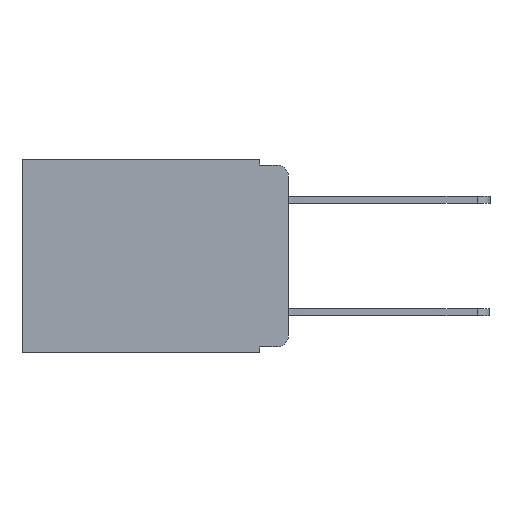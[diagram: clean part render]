
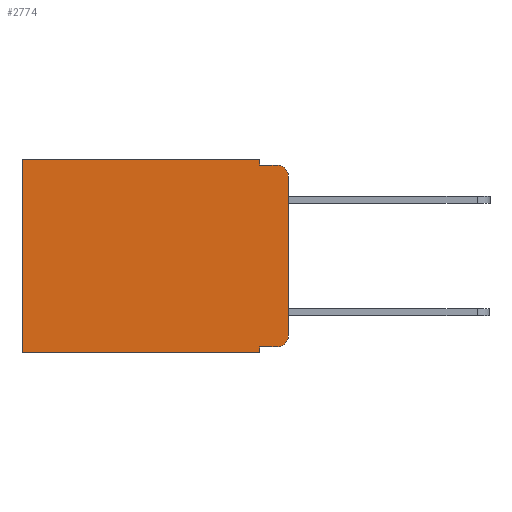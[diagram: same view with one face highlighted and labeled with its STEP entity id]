
A CAD part, left-side view. The second image highlights one B-rep face of the part: STEP entity #2774.
In plain terms, the highlighted planar face has unit normal (-1, 0, 0).
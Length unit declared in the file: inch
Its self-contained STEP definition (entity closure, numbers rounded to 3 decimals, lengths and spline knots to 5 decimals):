
#93 = LINE ( 'NONE', #8609, #8546 ) ;
#220 = VERTEX_POINT ( 'NONE', #7425 ) ;
#254 = VERTEX_POINT ( 'NONE', #4458 ) ;
#328 = ORIENTED_EDGE ( 'NONE', *, *, #1835, .T. ) ;
#384 = ORIENTED_EDGE ( 'NONE', *, *, #3540, .F. ) ;
#451 = CARTESIAN_POINT ( 'NONE',  ( 0.298, 0., 0. ) ) ;
#506 = ORIENTED_EDGE ( 'NONE', *, *, #4647, .T. ) ;
#510 = EDGE_CURVE ( 'NONE', #220, #4738, #2900, .T. ) ;
#689 = CARTESIAN_POINT ( 'NONE',  ( 0.298, 0.02, -0.313 ) ) ;
#1025 = VECTOR ( 'NONE', #7354, 39.37008 ) ;
#1147 = DIRECTION ( 'NONE',  ( 0., 0., -1. ) ) ;
#1182 = EDGE_CURVE ( 'NONE', #2240, #3297, #7693, .T. ) ;
#1307 = LINE ( 'NONE', #451, #9899 ) ;
#1418 = DIRECTION ( 'NONE',  ( 0., 1., 0. ) ) ;
#1739 = CARTESIAN_POINT ( 'NONE',  ( 0.298, 0., 0. ) ) ;
#1835 = EDGE_CURVE ( 'NONE', #220, #2240, #3275, .T. ) ;
#1979 = ORIENTED_EDGE ( 'NONE', *, *, #2464, .F. ) ;
#2043 = EDGE_CURVE ( 'NONE', #7304, #254, #1307, .T. ) ;
#2240 = VERTEX_POINT ( 'NONE', #3832 ) ;
#2464 = EDGE_CURVE ( 'NONE', #7281, #9256, #5841, .T. ) ;
#2553 = DIRECTION ( 'NONE',  ( -1., 0., 0. ) ) ;
#2678 = CARTESIAN_POINT ( 'NONE',  ( 0.298, 0.02, -0.03 ) ) ;
#2774 = ADVANCED_FACE ( 'NONE', ( #5222 ), #6593, .F. ) ;
#2776 = CARTESIAN_POINT ( 'NONE',  ( 0.298, 0.051, 0. ) ) ;
#2900 = LINE ( 'NONE', #2776, #7006 ) ;
#2901 = ORIENTED_EDGE ( 'NONE', *, *, #1182, .T. ) ;
#3275 = LINE ( 'NONE', #1739, #5734 ) ;
#3295 = ORIENTED_EDGE ( 'NONE', *, *, #4768, .T. ) ;
#3297 = VERTEX_POINT ( 'NONE', #9335 ) ;
#3540 = EDGE_CURVE ( 'NONE', #9256, #3297, #6058, .T. ) ;
#3547 = DIRECTION ( 'NONE',  ( 0., 0., -1. ) ) ;
#3669 = ORIENTED_EDGE ( 'NONE', *, *, #510, .F. ) ;
#3788 = LINE ( 'NONE', #9903, #9996 ) ;
#3792 = DIRECTION ( 'NONE',  ( 0., 0., -1. ) ) ;
#3832 = CARTESIAN_POINT ( 'NONE',  ( 0.298, 0.473, 0. ) ) ;
#4022 = AXIS2_PLACEMENT_3D ( 'NONE', #6584, #6695, #6679 ) ;
#4277 = AXIS2_PLACEMENT_3D ( 'NONE', #2678, #8287, #3547 ) ;
#4458 = CARTESIAN_POINT ( 'NONE',  ( 0.298, 0., -0.313 ) ) ;
#4515 = DIRECTION ( 'NONE',  ( 0., -1., 0. ) ) ;
#4647 = EDGE_CURVE ( 'NONE', #9297, #254, #9946, .T. ) ;
#4738 = VERTEX_POINT ( 'NONE', #9795 ) ;
#4768 = EDGE_CURVE ( 'NONE', #7281, #9297, #93, .T. ) ;
#4871 = CIRCLE ( 'NONE', #4277, 0.02 ) ;
#5222 = FACE_OUTER_BOUND ( 'NONE', #6805, .T. ) ;
#5734 = VECTOR ( 'NONE', #1418, 39.37008 ) ;
#5841 = LINE ( 'NONE', #8256, #7677 ) ;
#6058 = LINE ( 'NONE', #8070, #10085 ) ;
#6195 = CARTESIAN_POINT ( 'NONE',  ( 0.298, 0.051, -0.343 ) ) ;
#6229 = CARTESIAN_POINT ( 'NONE',  ( 0.298, 0.02, -0.333 ) ) ;
#6277 = VERTEX_POINT ( 'NONE', #8259 ) ;
#6316 = ORIENTED_EDGE ( 'NONE', *, *, #8549, .F. ) ;
#6498 = EDGE_CURVE ( 'NONE', #7304, #6277, #4871, .T. ) ;
#6584 = CARTESIAN_POINT ( 'NONE',  ( 0.298, 0., 0. ) ) ;
#6593 = PLANE ( 'NONE',  #4022 ) ;
#6679 = DIRECTION ( 'NONE',  ( 0., 0., -1. ) ) ;
#6695 = DIRECTION ( 'NONE',  ( 1., 0., 0. ) ) ;
#6805 = EDGE_LOOP ( 'NONE', ( #6945, #7990, #6316, #3669, #328, #2901, #384, #1979, #3295, #506 ) ) ;
#6836 = DIRECTION ( 'NONE',  ( 0., 0., -1. ) ) ;
#6945 = ORIENTED_EDGE ( 'NONE', *, *, #2043, .F. ) ;
#7006 = VECTOR ( 'NONE', #8233, 39.37008 ) ;
#7149 = AXIS2_PLACEMENT_3D ( 'NONE', #689, #2553, #1147 ) ;
#7281 = VERTEX_POINT ( 'NONE', #9181 ) ;
#7304 = VERTEX_POINT ( 'NONE', #9213 ) ;
#7354 = DIRECTION ( 'NONE',  ( 0., 0., -1. ) ) ;
#7425 = CARTESIAN_POINT ( 'NONE',  ( 0.298, 0.051, 0. ) ) ;
#7677 = VECTOR ( 'NONE', #3792, 39.37008 ) ;
#7693 = LINE ( 'NONE', #8067, #1025 ) ;
#7990 = ORIENTED_EDGE ( 'NONE', *, *, #6498, .T. ) ;
#8067 = CARTESIAN_POINT ( 'NONE',  ( 0.298, 0.473, 0. ) ) ;
#8070 = CARTESIAN_POINT ( 'NONE',  ( 0.298, 0., -0.343 ) ) ;
#8233 = DIRECTION ( 'NONE',  ( 0., 0., -1. ) ) ;
#8256 = CARTESIAN_POINT ( 'NONE',  ( 0.298, 0.051, 0. ) ) ;
#8259 = CARTESIAN_POINT ( 'NONE',  ( 0.298, 0.02, -0.01 ) ) ;
#8287 = DIRECTION ( 'NONE',  ( -1., 0., 0. ) ) ;
#8475 = DIRECTION ( 'NONE',  ( 0., -1., 0. ) ) ;
#8546 = VECTOR ( 'NONE', #8475, 39.37008 ) ;
#8549 = EDGE_CURVE ( 'NONE', #4738, #6277, #3788, .T. ) ;
#8589 = DIRECTION ( 'NONE',  ( 0., 1., 0. ) ) ;
#8609 = CARTESIAN_POINT ( 'NONE',  ( 0.298, 0.051, -0.333 ) ) ;
#9181 = CARTESIAN_POINT ( 'NONE',  ( 0.298, 0.051, -0.333 ) ) ;
#9213 = CARTESIAN_POINT ( 'NONE',  ( 0.298, 0., -0.03 ) ) ;
#9256 = VERTEX_POINT ( 'NONE', #6195 ) ;
#9297 = VERTEX_POINT ( 'NONE', #6229 ) ;
#9335 = CARTESIAN_POINT ( 'NONE',  ( 0.298, 0.473, -0.343 ) ) ;
#9795 = CARTESIAN_POINT ( 'NONE',  ( 0.298, 0.051, -0.01 ) ) ;
#9899 = VECTOR ( 'NONE', #6836, 39.37008 ) ;
#9903 = CARTESIAN_POINT ( 'NONE',  ( 0.298, 0.051, -0.01 ) ) ;
#9946 = CIRCLE ( 'NONE', #7149, 0.02 ) ;
#9996 = VECTOR ( 'NONE', #4515, 39.37008 ) ;
#10085 = VECTOR ( 'NONE', #8589, 39.37008 ) ;
